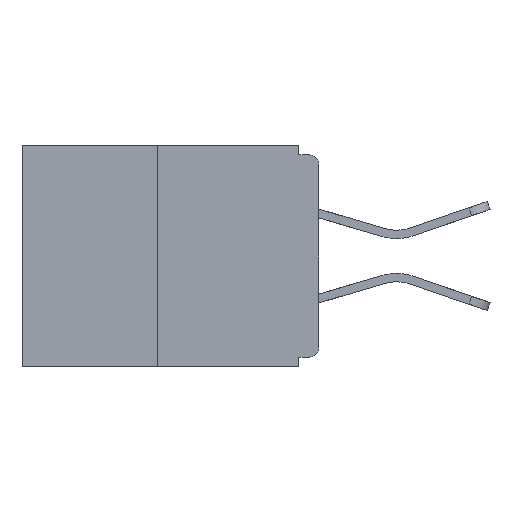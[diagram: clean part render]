
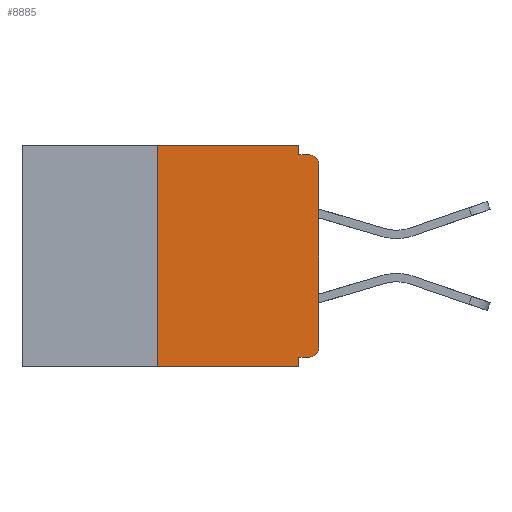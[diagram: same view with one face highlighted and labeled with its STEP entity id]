
A CAD part, left-side view. The second image highlights one B-rep face of the part: STEP entity #8885.
In plain terms, the highlighted planar face has unit normal (-1, 0, 0).
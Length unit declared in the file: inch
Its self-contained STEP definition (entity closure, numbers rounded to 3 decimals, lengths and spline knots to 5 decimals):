
#862 = FACE_OUTER_BOUND ( 'NONE', #11021, .T. ) ;
#1319 = CARTESIAN_POINT ( 'NONE',  ( 0., 0.46, -0.343 ) ) ;
#1418 = CARTESIAN_POINT ( 'NONE',  ( 0., 0.015, -0.313 ) ) ;
#2059 = ORIENTED_EDGE ( 'NONE', *, *, #2733, .F. ) ;
#2350 = VECTOR ( 'NONE', #10739, 39.37008 ) ;
#2358 = VERTEX_POINT ( 'NONE', #10720 ) ;
#2593 = DIRECTION ( 'NONE',  ( 0., 0., -1. ) ) ;
#2611 = CARTESIAN_POINT ( 'NONE',  ( 0., 0.46, 0. ) ) ;
#2733 = EDGE_CURVE ( 'NONE', #9764, #13870, #16557, .T. ) ;
#2772 = VECTOR ( 'NONE', #10990, 39.37008 ) ;
#3037 = EDGE_CURVE ( 'NONE', #13870, #13273, #3422, .T. ) ;
#3213 = EDGE_CURVE ( 'NONE', #17386, #9764, #8229, .T. ) ;
#3239 = EDGE_CURVE ( 'NONE', #5835, #11007, #8690, .T. ) ;
#3359 = DIRECTION ( 'NONE',  ( 0., 0., -1. ) ) ;
#3422 = LINE ( 'NONE', #15038, #2772 ) ;
#3431 = LINE ( 'NONE', #5814, #5518 ) ;
#4667 = LINE ( 'NONE', #10099, #10375 ) ;
#4918 = ORIENTED_EDGE ( 'NONE', *, *, #3037, .F. ) ;
#5034 = CARTESIAN_POINT ( 'NONE',  ( 0., 0.25, 0. ) ) ;
#5243 = DIRECTION ( 'NONE',  ( -1., 0., 0. ) ) ;
#5518 = VECTOR ( 'NONE', #3359, 39.37008 ) ;
#5527 = ORIENTED_EDGE ( 'NONE', *, *, #6568, .T. ) ;
#5660 = LINE ( 'NONE', #5676, #15220 ) ;
#5676 = CARTESIAN_POINT ( 'NONE',  ( 0., 0., 0. ) ) ;
#5814 = CARTESIAN_POINT ( 'NONE',  ( 0., 0.031, -0.343 ) ) ;
#5835 = VERTEX_POINT ( 'NONE', #10604 ) ;
#5890 = DIRECTION ( 'NONE',  ( 0., 0., -1. ) ) ;
#6124 = CARTESIAN_POINT ( 'NONE',  ( 0., 0.015, -0.328 ) ) ;
#6479 = ORIENTED_EDGE ( 'NONE', *, *, #9139, .T. ) ;
#6568 = EDGE_CURVE ( 'NONE', #10916, #10500, #9954, .T. ) ;
#6570 = DIRECTION ( 'NONE',  ( 0., 0., -1. ) ) ;
#7192 = CIRCLE ( 'NONE', #12585, 0.015 ) ;
#7968 = DIRECTION ( 'NONE',  ( 1., 0., 0. ) ) ;
#8023 = EDGE_CURVE ( 'NONE', #2358, #13273, #7192, .T. ) ;
#8109 = EDGE_CURVE ( 'NONE', #10916, #11293, #4667, .T. ) ;
#8143 = CARTESIAN_POINT ( 'NONE',  ( 0., 0., -0.313 ) ) ;
#8229 = LINE ( 'NONE', #2611, #17350 ) ;
#8295 = LINE ( 'NONE', #16778, #16798 ) ;
#8657 = DIRECTION ( 'NONE',  ( 0., 0., 1. ) ) ;
#8690 = LINE ( 'NONE', #1319, #2350 ) ;
#8885 = ADVANCED_FACE ( 'NONE', ( #862 ), #12145, .F. ) ;
#9139 = EDGE_CURVE ( 'NONE', #10500, #2358, #5660, .T. ) ;
#9309 = ORIENTED_EDGE ( 'NONE', *, *, #10605, .F. ) ;
#9502 = DIRECTION ( 'NONE',  ( 0., -1., 0. ) ) ;
#9537 = VECTOR ( 'NONE', #17110, 39.37008 ) ;
#9764 = VERTEX_POINT ( 'NONE', #13968 ) ;
#9954 = CIRCLE ( 'NONE', #11746, 0.015 ) ;
#10041 = DIRECTION ( 'NONE',  ( 0., 1., 0. ) ) ;
#10099 = CARTESIAN_POINT ( 'NONE',  ( 0., 0., -0.328 ) ) ;
#10374 = CARTESIAN_POINT ( 'NONE',  ( 0., 0.031, -0.015 ) ) ;
#10375 = VECTOR ( 'NONE', #10041, 39.37008 ) ;
#10500 = VERTEX_POINT ( 'NONE', #8143 ) ;
#10604 = CARTESIAN_POINT ( 'NONE',  ( 0., 0.25, -0.343 ) ) ;
#10605 = EDGE_CURVE ( 'NONE', #11293, #11007, #3431, .T. ) ;
#10720 = CARTESIAN_POINT ( 'NONE',  ( 0., 0., -0.03 ) ) ;
#10739 = DIRECTION ( 'NONE',  ( 0., -1., 0. ) ) ;
#10765 = CARTESIAN_POINT ( 'NONE',  ( 0., 0.46, 0. ) ) ;
#10876 = ORIENTED_EDGE ( 'NONE', *, *, #8023, .T. ) ;
#10916 = VERTEX_POINT ( 'NONE', #6124 ) ;
#10990 = DIRECTION ( 'NONE',  ( 0., -1., 0. ) ) ;
#11007 = VERTEX_POINT ( 'NONE', #13327 ) ;
#11021 = EDGE_LOOP ( 'NONE', ( #16201, #16729, #14548, #9309, #15917, #5527, #6479, #10876, #4918, #2059 ) ) ;
#11293 = VERTEX_POINT ( 'NONE', #12220 ) ;
#11501 = CARTESIAN_POINT ( 'NONE',  ( 0., 0.031, 0. ) ) ;
#11746 = AXIS2_PLACEMENT_3D ( 'NONE', #1418, #5243, #2593 ) ;
#12145 = PLANE ( 'NONE',  #17028 ) ;
#12220 = CARTESIAN_POINT ( 'NONE',  ( 0., 0.031, -0.328 ) ) ;
#12585 = AXIS2_PLACEMENT_3D ( 'NONE', #13963, #15335, #5890 ) ;
#13273 = VERTEX_POINT ( 'NONE', #14529 ) ;
#13327 = CARTESIAN_POINT ( 'NONE',  ( 0., 0.031, -0.343 ) ) ;
#13870 = VERTEX_POINT ( 'NONE', #10374 ) ;
#13963 = CARTESIAN_POINT ( 'NONE',  ( 0., 0.015, -0.03 ) ) ;
#13968 = CARTESIAN_POINT ( 'NONE',  ( 0., 0.031, 0. ) ) ;
#14529 = CARTESIAN_POINT ( 'NONE',  ( 0., 0.015, -0.015 ) ) ;
#14548 = ORIENTED_EDGE ( 'NONE', *, *, #3239, .T. ) ;
#15038 = CARTESIAN_POINT ( 'NONE',  ( 0., 0., -0.015 ) ) ;
#15099 = EDGE_CURVE ( 'NONE', #5835, #17386, #8295, .T. ) ;
#15220 = VECTOR ( 'NONE', #16532, 39.37008 ) ;
#15335 = DIRECTION ( 'NONE',  ( -1., 0., 0. ) ) ;
#15917 = ORIENTED_EDGE ( 'NONE', *, *, #8109, .F. ) ;
#16201 = ORIENTED_EDGE ( 'NONE', *, *, #3213, .F. ) ;
#16532 = DIRECTION ( 'NONE',  ( 0., 0., 1. ) ) ;
#16557 = LINE ( 'NONE', #11501, #9537 ) ;
#16729 = ORIENTED_EDGE ( 'NONE', *, *, #15099, .F. ) ;
#16778 = CARTESIAN_POINT ( 'NONE',  ( 0., 0.25, 0. ) ) ;
#16798 = VECTOR ( 'NONE', #8657, 39.37008 ) ;
#17028 = AXIS2_PLACEMENT_3D ( 'NONE', #10765, #7968, #6570 ) ;
#17110 = DIRECTION ( 'NONE',  ( 0., 0., -1. ) ) ;
#17350 = VECTOR ( 'NONE', #9502, 39.37008 ) ;
#17386 = VERTEX_POINT ( 'NONE', #5034 ) ;
